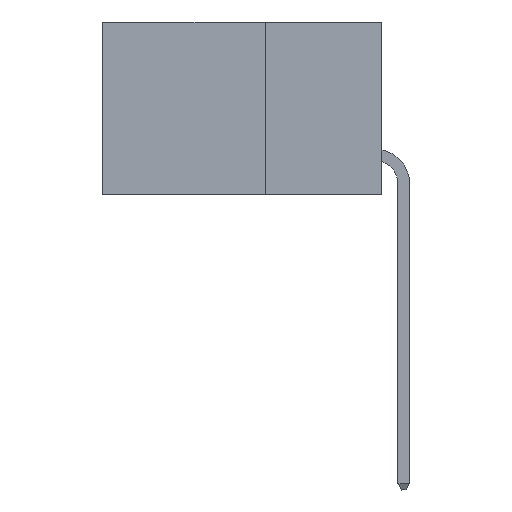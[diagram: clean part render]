
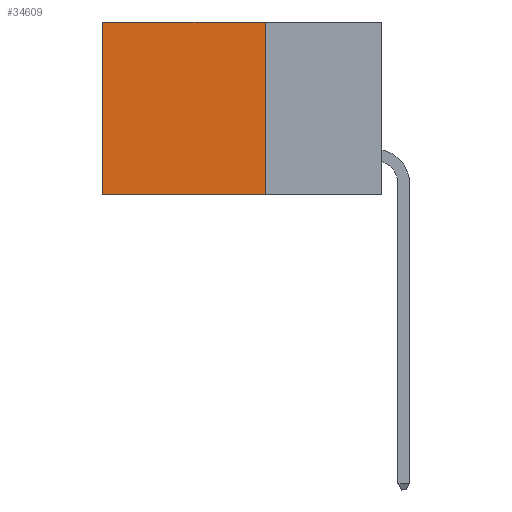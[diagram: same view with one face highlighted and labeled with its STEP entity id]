
A CAD part, left-side view. The second image highlights one B-rep face of the part: STEP entity #34609.
In plain terms, the highlighted planar face has unit normal (-1, 0, 0).
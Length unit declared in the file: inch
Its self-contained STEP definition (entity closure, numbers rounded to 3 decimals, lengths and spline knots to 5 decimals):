
#1475 = VERTEX_POINT ( 'NONE', #22877 ) ;
#1805 = DIRECTION ( 'NONE',  ( 0., 0., -1. ) ) ;
#2208 = DIRECTION ( 'NONE',  ( 0., 1., 0. ) ) ;
#3505 = CARTESIAN_POINT ( 'NONE',  ( 0.2875, 0.6, 0. ) ) ;
#6833 = LINE ( 'NONE', #3505, #17356 ) ;
#8189 = VERTEX_POINT ( 'NONE', #15812 ) ;
#8474 = EDGE_CURVE ( 'NONE', #43449, #1475, #18805, .T. ) ;
#9868 = FACE_OUTER_BOUND ( 'NONE', #35084, .T. ) ;
#9917 = VECTOR ( 'NONE', #1805, 39.37008 ) ;
#10659 = VECTOR ( 'NONE', #2208, 39.37008 ) ;
#11510 = CARTESIAN_POINT ( 'NONE',  ( 0.2875, 0.6, 0. ) ) ;
#12901 = DIRECTION ( 'NONE',  ( 0., 1., 0. ) ) ;
#13326 = ORIENTED_EDGE ( 'NONE', *, *, #8474, .F. ) ;
#14210 = DIRECTION ( 'NONE',  ( 0., 0., -1. ) ) ;
#15157 = CARTESIAN_POINT ( 'NONE',  ( 0.2875, 0.25, -0.37 ) ) ;
#15812 = CARTESIAN_POINT ( 'NONE',  ( 0.2875, 0.25, 0. ) ) ;
#16467 = EDGE_CURVE ( 'NONE', #8189, #43449, #28715, .T. ) ;
#17356 = VECTOR ( 'NONE', #14210, 39.37008 ) ;
#17892 = ORIENTED_EDGE ( 'NONE', *, *, #42969, .T. ) ;
#18266 = DIRECTION ( 'NONE',  ( 1., 0., 0. ) ) ;
#18731 = PLANE ( 'NONE',  #24696 ) ;
#18805 = LINE ( 'NONE', #27176, #43794 ) ;
#20936 = ORIENTED_EDGE ( 'NONE', *, *, #16467, .F. ) ;
#22877 = CARTESIAN_POINT ( 'NONE',  ( 0.2875, 0.6, -0.37 ) ) ;
#23230 = CARTESIAN_POINT ( 'NONE',  ( 0.2875, 0.25, 0. ) ) ;
#24696 = AXIS2_PLACEMENT_3D ( 'NONE', #35918, #18266, #33576 ) ;
#27176 = CARTESIAN_POINT ( 'NONE',  ( 0.2875, 0.25, -0.37 ) ) ;
#28715 = LINE ( 'NONE', #37098, #9917 ) ;
#30953 = VERTEX_POINT ( 'NONE', #11510 ) ;
#32785 = LINE ( 'NONE', #23230, #10659 ) ;
#33576 = DIRECTION ( 'NONE',  ( 0., 0., -1. ) ) ;
#34609 = ADVANCED_FACE ( 'NONE', ( #9868 ), #18731, .F. ) ;
#35084 = EDGE_LOOP ( 'NONE', ( #39726, #13326, #20936, #17892 ) ) ;
#35918 = CARTESIAN_POINT ( 'NONE',  ( 0.2875, 0.25, 0. ) ) ;
#37098 = CARTESIAN_POINT ( 'NONE',  ( 0.2875, 0.25, 0. ) ) ;
#37109 = EDGE_CURVE ( 'NONE', #30953, #1475, #6833, .T. ) ;
#39726 = ORIENTED_EDGE ( 'NONE', *, *, #37109, .T. ) ;
#42969 = EDGE_CURVE ( 'NONE', #8189, #30953, #32785, .T. ) ;
#43449 = VERTEX_POINT ( 'NONE', #15157 ) ;
#43794 = VECTOR ( 'NONE', #12901, 39.37008 ) ;
